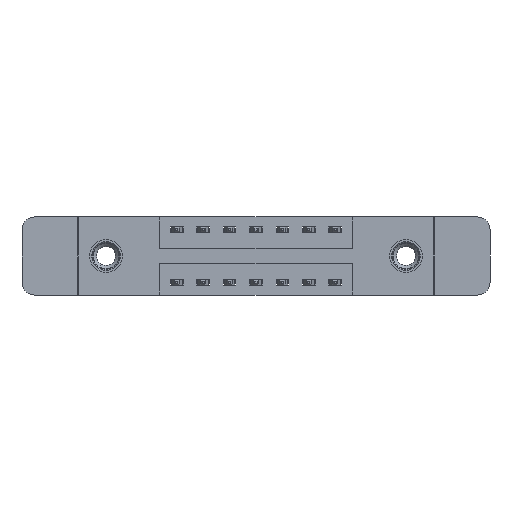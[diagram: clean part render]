
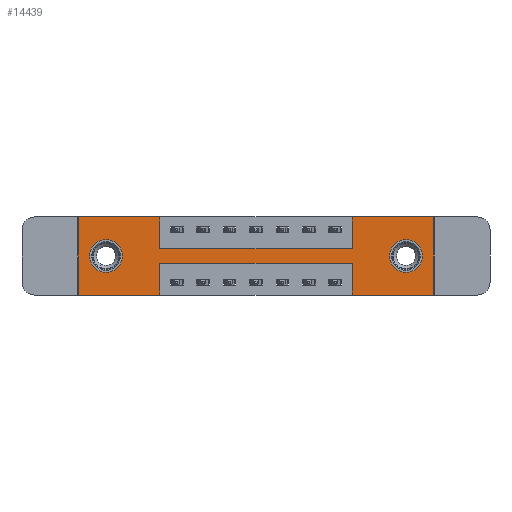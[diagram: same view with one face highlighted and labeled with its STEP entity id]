
A CAD part, front view. The second image highlights one B-rep face of the part: STEP entity #14439.
In plain terms, the highlighted planar face has unit normal (0, -1, 0).
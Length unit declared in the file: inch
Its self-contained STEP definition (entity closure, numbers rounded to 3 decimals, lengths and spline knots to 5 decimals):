
#29 = FACE_OUTER_BOUND ( 'NONE', #8252, .T. ) ;
#108 = DIRECTION ( 'NONE',  ( 0., 0., -1. ) ) ;
#109 = VECTOR ( 'NONE', #12804, 39.37008 ) ;
#563 = VECTOR ( 'NONE', #7209, 39.37008 ) ;
#700 = ORIENTED_EDGE ( 'NONE', *, *, #1207, .F. ) ;
#752 = VERTEX_POINT ( 'NONE', #7595 ) ;
#792 = LINE ( 'NONE', #3185, #2693 ) ;
#837 = AXIS2_PLACEMENT_3D ( 'NONE', #13937, #3818, #12876 ) ;
#1026 = ORIENTED_EDGE ( 'NONE', *, *, #11171, .F. ) ;
#1045 = ORIENTED_EDGE ( 'NONE', *, *, #2225, .T. ) ;
#1130 = VERTEX_POINT ( 'NONE', #6211 ) ;
#1145 = CARTESIAN_POINT ( 'NONE',  ( 0.3875, 0., 0. ) ) ;
#1207 = EDGE_CURVE ( 'NONE', #10263, #8938, #3774, .T. ) ;
#1379 = CARTESIAN_POINT ( 'NONE',  ( 0., 0., -0.37 ) ) ;
#1615 = LINE ( 'NONE', #14237, #3880 ) ;
#1707 = DIRECTION ( 'NONE',  ( 0., 0., 1. ) ) ;
#1824 = EDGE_CURVE ( 'NONE', #4052, #5593, #792, .T. ) ;
#1842 = LINE ( 'NONE', #12496, #10417 ) ;
#1851 = DIRECTION ( 'NONE',  ( 1., 0., 0. ) ) ;
#1919 = LINE ( 'NONE', #5279, #9507 ) ;
#2202 = DIRECTION ( 'NONE',  ( 0., -1., 0. ) ) ;
#2225 = EDGE_CURVE ( 'NONE', #11091, #7053, #9558, .T. ) ;
#2264 = LINE ( 'NONE', #1145, #563 ) ;
#2279 = FACE_BOUND ( 'NONE', #5126, .T. ) ;
#2510 = VECTOR ( 'NONE', #9842, 39.37008 ) ;
#2545 = VERTEX_POINT ( 'NONE', #9532 ) ;
#2649 = EDGE_CURVE ( 'NONE', #12276, #14501, #12093, .T. ) ;
#2661 = ORIENTED_EDGE ( 'NONE', *, *, #1824, .F. ) ;
#2693 = VECTOR ( 'NONE', #13336, 39.37008 ) ;
#2728 = LINE ( 'NONE', #8200, #14132 ) ;
#2903 = CARTESIAN_POINT ( 'NONE',  ( 1.2975, 0., -0.22 ) ) ;
#2981 = VECTOR ( 'NONE', #7213, 39.37008 ) ;
#3114 = DIRECTION ( 'NONE',  ( 0., 0., 1. ) ) ;
#3185 = CARTESIAN_POINT ( 'NONE',  ( 0., 0., -0.37 ) ) ;
#3271 = PLANE ( 'NONE',  #3759 ) ;
#3342 = CARTESIAN_POINT ( 'NONE',  ( 1.5525, 0., -0.185 ) ) ;
#3410 = ORIENTED_EDGE ( 'NONE', *, *, #7927, .F. ) ;
#3418 = DIRECTION ( 'NONE',  ( 0., 0., -1. ) ) ;
#3673 = ORIENTED_EDGE ( 'NONE', *, *, #4178, .T. ) ;
#3708 = CARTESIAN_POINT ( 'NONE',  ( 0.3875, 0., -0.37 ) ) ;
#3759 = AXIS2_PLACEMENT_3D ( 'NONE', #13563, #2202, #3418 ) ;
#3774 = LINE ( 'NONE', #6131, #6517 ) ;
#3818 = DIRECTION ( 'NONE',  ( 0., 1., 0. ) ) ;
#3880 = VECTOR ( 'NONE', #6016, 39.37008 ) ;
#4039 = ORIENTED_EDGE ( 'NONE', *, *, #14541, .F. ) ;
#4052 = VERTEX_POINT ( 'NONE', #11406 ) ;
#4178 = EDGE_CURVE ( 'NONE', #7337, #752, #12639, .T. ) ;
#4298 = CARTESIAN_POINT ( 'NONE',  ( 0., 0., -0.37 ) ) ;
#4317 = DIRECTION ( 'NONE',  ( 0., 1., 0. ) ) ;
#4614 = DIRECTION ( 'NONE',  ( 0., 0., 1. ) ) ;
#4629 = DIRECTION ( 'NONE',  ( 0., 0., -1. ) ) ;
#4649 = CARTESIAN_POINT ( 'NONE',  ( 0.3875, 0., 0. ) ) ;
#4684 = LINE ( 'NONE', #5683, #14758 ) ;
#5126 = EDGE_LOOP ( 'NONE', ( #8647, #1045 ) ) ;
#5207 = ORIENTED_EDGE ( 'NONE', *, *, #13183, .T. ) ;
#5279 = CARTESIAN_POINT ( 'NONE',  ( 0., 0., 0. ) ) ;
#5447 = CIRCLE ( 'NONE', #837, 0.078 ) ;
#5558 = CARTESIAN_POINT ( 'NONE',  ( 0., 0., 0. ) ) ;
#5593 = VERTEX_POINT ( 'NONE', #8937 ) ;
#5683 = CARTESIAN_POINT ( 'NONE',  ( 0., 0., 0. ) ) ;
#5846 = DIRECTION ( 'NONE',  ( 0., 1., 0. ) ) ;
#6016 = DIRECTION ( 'NONE',  ( 1., 0., 0. ) ) ;
#6108 = ORIENTED_EDGE ( 'NONE', *, *, #11788, .F. ) ;
#6131 = CARTESIAN_POINT ( 'NONE',  ( 0.3875, 0., -0.22 ) ) ;
#6147 = LINE ( 'NONE', #12707, #2981 ) ;
#6150 = CARTESIAN_POINT ( 'NONE',  ( 1.5525, 0., -0.107 ) ) ;
#6211 = CARTESIAN_POINT ( 'NONE',  ( 1.2975, 0., 0. ) ) ;
#6278 = ORIENTED_EDGE ( 'NONE', *, *, #12275, .F. ) ;
#6517 = VECTOR ( 'NONE', #8473, 39.37008 ) ;
#6595 = EDGE_CURVE ( 'NONE', #10490, #14158, #1615, .T. ) ;
#6731 = ORIENTED_EDGE ( 'NONE', *, *, #6595, .F. ) ;
#7053 = VERTEX_POINT ( 'NONE', #6150 ) ;
#7209 = DIRECTION ( 'NONE',  ( 0., 0., -1. ) ) ;
#7213 = DIRECTION ( 'NONE',  ( 0., 0., -1. ) ) ;
#7337 = VERTEX_POINT ( 'NONE', #11772 ) ;
#7595 = CARTESIAN_POINT ( 'NONE',  ( 0.1325, 0., -0.263 ) ) ;
#7596 = DIRECTION ( 'NONE',  ( 0., 0., -1. ) ) ;
#7783 = DIRECTION ( 'NONE',  ( 0., 1., 0. ) ) ;
#7831 = LINE ( 'NONE', #11363, #9764 ) ;
#7889 = AXIS2_PLACEMENT_3D ( 'NONE', #8725, #4317, #7596 ) ;
#7908 = DIRECTION ( 'NONE',  ( 0., 0., 1. ) ) ;
#7927 = EDGE_CURVE ( 'NONE', #13222, #1130, #1842, .T. ) ;
#8058 = EDGE_CURVE ( 'NONE', #7053, #11091, #14746, .T. ) ;
#8200 = CARTESIAN_POINT ( 'NONE',  ( 0.3875, 0., -0.37 ) ) ;
#8252 = EDGE_LOOP ( 'NONE', ( #4039, #700, #13064, #2661, #6278, #6108, #3410, #10039, #1026, #6731, #9714, #11804 ) ) ;
#8386 = VERTEX_POINT ( 'NONE', #9862 ) ;
#8473 = DIRECTION ( 'NONE',  ( -1., 0., 0. ) ) ;
#8560 = EDGE_CURVE ( 'NONE', #14501, #10490, #4684, .T. ) ;
#8647 = ORIENTED_EDGE ( 'NONE', *, *, #8058, .T. ) ;
#8725 = CARTESIAN_POINT ( 'NONE',  ( 1.5525, 0., -0.185 ) ) ;
#8844 = CARTESIAN_POINT ( 'NONE',  ( 0.1325, 0., -0.185 ) ) ;
#8937 = CARTESIAN_POINT ( 'NONE',  ( 1.2975, 0., -0.37 ) ) ;
#8938 = VERTEX_POINT ( 'NONE', #14492 ) ;
#9243 = CARTESIAN_POINT ( 'NONE',  ( 1.5525, 0., -0.263 ) ) ;
#9414 = CARTESIAN_POINT ( 'NONE',  ( 1.2975, 0., -0.15 ) ) ;
#9507 = VECTOR ( 'NONE', #1851, 39.37008 ) ;
#9532 = CARTESIAN_POINT ( 'NONE',  ( 0.3875, 0., -0.15 ) ) ;
#9558 = CIRCLE ( 'NONE', #7889, 0.078 ) ;
#9714 = ORIENTED_EDGE ( 'NONE', *, *, #8560, .F. ) ;
#9764 = VECTOR ( 'NONE', #7908, 39.37008 ) ;
#9842 = DIRECTION ( 'NONE',  ( -1., 0., 0. ) ) ;
#9862 = CARTESIAN_POINT ( 'NONE',  ( 1.685, 0., 0. ) ) ;
#10008 = AXIS2_PLACEMENT_3D ( 'NONE', #8844, #7783, #1707 ) ;
#10039 = ORIENTED_EDGE ( 'NONE', *, *, #12957, .F. ) ;
#10263 = VERTEX_POINT ( 'NONE', #2903 ) ;
#10417 = VECTOR ( 'NONE', #3114, 39.37008 ) ;
#10490 = VERTEX_POINT ( 'NONE', #5558 ) ;
#11091 = VERTEX_POINT ( 'NONE', #9243 ) ;
#11171 = EDGE_CURVE ( 'NONE', #14158, #2545, #2264, .T. ) ;
#11363 = CARTESIAN_POINT ( 'NONE',  ( 1.2975, 0., -0.37 ) ) ;
#11406 = CARTESIAN_POINT ( 'NONE',  ( 1.685, 0., -0.37 ) ) ;
#11772 = CARTESIAN_POINT ( 'NONE',  ( 0.1325, 0., -0.107 ) ) ;
#11788 = EDGE_CURVE ( 'NONE', #1130, #8386, #1919, .T. ) ;
#11804 = ORIENTED_EDGE ( 'NONE', *, *, #2649, .F. ) ;
#12093 = LINE ( 'NONE', #4298, #2510 ) ;
#12169 = EDGE_CURVE ( 'NONE', #5593, #10263, #7831, .T. ) ;
#12275 = EDGE_CURVE ( 'NONE', #8386, #4052, #6147, .T. ) ;
#12276 = VERTEX_POINT ( 'NONE', #3708 ) ;
#12496 = CARTESIAN_POINT ( 'NONE',  ( 1.2975, 0., 0. ) ) ;
#12639 = CIRCLE ( 'NONE', #10008, 0.078 ) ;
#12707 = CARTESIAN_POINT ( 'NONE',  ( 1.685, 0., 0. ) ) ;
#12804 = DIRECTION ( 'NONE',  ( 1., 0., 0. ) ) ;
#12876 = DIRECTION ( 'NONE',  ( 0., 0., 1. ) ) ;
#12957 = EDGE_CURVE ( 'NONE', #2545, #13222, #13040, .T. ) ;
#12970 = EDGE_LOOP ( 'NONE', ( #3673, #5207 ) ) ;
#13040 = LINE ( 'NONE', #13869, #109 ) ;
#13064 = ORIENTED_EDGE ( 'NONE', *, *, #12169, .F. ) ;
#13183 = EDGE_CURVE ( 'NONE', #752, #7337, #5447, .T. ) ;
#13222 = VERTEX_POINT ( 'NONE', #9414 ) ;
#13336 = DIRECTION ( 'NONE',  ( -1., 0., 0. ) ) ;
#13563 = CARTESIAN_POINT ( 'NONE',  ( 0., 0., -0.37 ) ) ;
#13711 = FACE_BOUND ( 'NONE', #12970, .T. ) ;
#13794 = AXIS2_PLACEMENT_3D ( 'NONE', #3342, #5846, #4629 ) ;
#13869 = CARTESIAN_POINT ( 'NONE',  ( 0.3875, 0., -0.15 ) ) ;
#13937 = CARTESIAN_POINT ( 'NONE',  ( 0.1325, 0., -0.185 ) ) ;
#14132 = VECTOR ( 'NONE', #108, 39.37008 ) ;
#14158 = VERTEX_POINT ( 'NONE', #4649 ) ;
#14237 = CARTESIAN_POINT ( 'NONE',  ( 0., 0., 0. ) ) ;
#14439 = ADVANCED_FACE ( 'NONE', ( #2279, #13711, #29 ), #3271, .T. ) ;
#14492 = CARTESIAN_POINT ( 'NONE',  ( 0.3875, 0., -0.22 ) ) ;
#14501 = VERTEX_POINT ( 'NONE', #1379 ) ;
#14541 = EDGE_CURVE ( 'NONE', #8938, #12276, #2728, .T. ) ;
#14746 = CIRCLE ( 'NONE', #13794, 0.078 ) ;
#14758 = VECTOR ( 'NONE', #4614, 39.37008 ) ;
